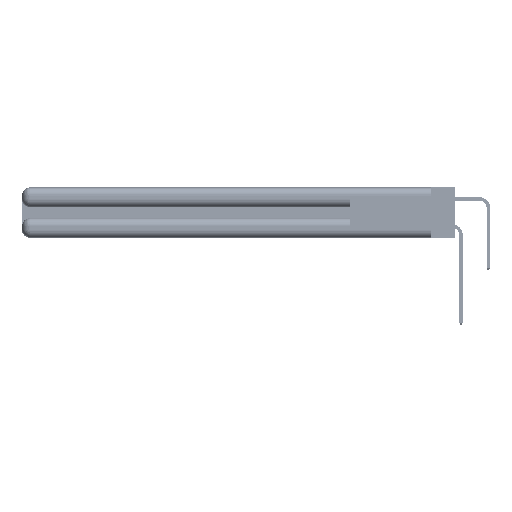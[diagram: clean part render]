
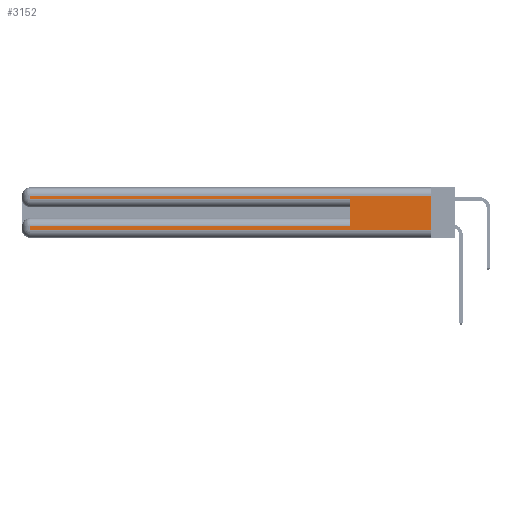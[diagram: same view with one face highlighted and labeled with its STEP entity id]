
A CAD part, left-side view. The second image highlights one B-rep face of the part: STEP entity #3152.
In plain terms, the highlighted planar face has unit normal (-1, 0, 0).
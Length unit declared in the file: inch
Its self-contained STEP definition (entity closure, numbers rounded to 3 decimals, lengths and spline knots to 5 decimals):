
#1266 = CARTESIAN_POINT ( 'NONE',  ( 0., 0., 0.085 ) ) ;
#1455 = VERTEX_POINT ( 'NONE', #17711 ) ;
#2959 = ORIENTED_EDGE ( 'NONE', *, *, #5836, .T. ) ;
#3152 = ADVANCED_FACE ( 'NONE', ( #15812 ), #12290, .F. ) ;
#4773 = ORIENTED_EDGE ( 'NONE', *, *, #14614, .T. ) ;
#5836 = EDGE_CURVE ( 'NONE', #51356, #11922, #20394, .T. ) ;
#5953 = VERTEX_POINT ( 'NONE', #56680 ) ;
#6262 = LINE ( 'NONE', #46348, #47936 ) ;
#6384 = LINE ( 'NONE', #8301, #53842 ) ;
#6420 = DIRECTION ( 'NONE',  ( 0., -1., 0. ) ) ;
#6842 = CARTESIAN_POINT ( 'NONE',  ( 0., 0., 0.06 ) ) ;
#8033 = ORIENTED_EDGE ( 'NONE', *, *, #21354, .F. ) ;
#8156 = ORIENTED_EDGE ( 'NONE', *, *, #21799, .F. ) ;
#8167 = AXIS2_PLACEMENT_3D ( 'NONE', #44431, #55079, #16702 ) ;
#8301 = CARTESIAN_POINT ( 'NONE',  ( 0., 0.6, 0.145 ) ) ;
#9534 = DIRECTION ( 'NONE',  ( 0., 1., 0. ) ) ;
#9538 = CARTESIAN_POINT ( 'NONE',  ( 0., 2.94, 0.37 ) ) ;
#11922 = VERTEX_POINT ( 'NONE', #40987 ) ;
#12290 = PLANE ( 'NONE',  #8167 ) ;
#13290 = LINE ( 'NONE', #29374, #29796 ) ;
#13654 = LINE ( 'NONE', #41084, #37311 ) ;
#14614 = EDGE_CURVE ( 'NONE', #1455, #5953, #6262, .T. ) ;
#15181 = LINE ( 'NONE', #9538, #19472 ) ;
#15812 = FACE_OUTER_BOUND ( 'NONE', #48353, .T. ) ;
#16702 = DIRECTION ( 'NONE',  ( 0., 0., -1. ) ) ;
#17130 = VECTOR ( 'NONE', #6420, 39.37008 ) ;
#17711 = CARTESIAN_POINT ( 'NONE',  ( 0., 0., 0.31 ) ) ;
#19472 = VECTOR ( 'NONE', #55698, 39.37008 ) ;
#19954 = VERTEX_POINT ( 'NONE', #22687 ) ;
#20394 = LINE ( 'NONE', #1266, #59277 ) ;
#20502 = CARTESIAN_POINT ( 'NONE',  ( 0., 0., 0.37 ) ) ;
#21083 = EDGE_CURVE ( 'NONE', #11922, #50777, #13654, .T. ) ;
#21354 = EDGE_CURVE ( 'NONE', #1455, #52335, #27208, .T. ) ;
#21799 = EDGE_CURVE ( 'NONE', #51356, #19954, #6384, .T. ) ;
#22687 = CARTESIAN_POINT ( 'NONE',  ( 0., 0.6, 0.285 ) ) ;
#26573 = VERTEX_POINT ( 'NONE', #51967 ) ;
#27208 = LINE ( 'NONE', #20502, #56703 ) ;
#28840 = EDGE_CURVE ( 'NONE', #5953, #26573, #15181, .T. ) ;
#29374 = CARTESIAN_POINT ( 'NONE',  ( 0., 0., 0.285 ) ) ;
#29796 = VECTOR ( 'NONE', #56725, 39.37008 ) ;
#31964 = ORIENTED_EDGE ( 'NONE', *, *, #21083, .T. ) ;
#32956 = EDGE_CURVE ( 'NONE', #26573, #19954, #13290, .T. ) ;
#33607 = LINE ( 'NONE', #33874, #17130 ) ;
#33874 = CARTESIAN_POINT ( 'NONE',  ( 0., 0., 0.06 ) ) ;
#33948 = DIRECTION ( 'NONE',  ( 0., 0., -1. ) ) ;
#37311 = VECTOR ( 'NONE', #41678, 39.37008 ) ;
#39554 = CARTESIAN_POINT ( 'NONE',  ( 0., 2.94, 0.06 ) ) ;
#39597 = ORIENTED_EDGE ( 'NONE', *, *, #32956, .T. ) ;
#39686 = CARTESIAN_POINT ( 'NONE',  ( 0., 0.6, 0.085 ) ) ;
#40418 = DIRECTION ( 'NONE',  ( 0., 0., 1. ) ) ;
#40987 = CARTESIAN_POINT ( 'NONE',  ( 0., 2.94, 0.085 ) ) ;
#41084 = CARTESIAN_POINT ( 'NONE',  ( 0., 2.94, 0.37 ) ) ;
#41678 = DIRECTION ( 'NONE',  ( 0., 0., -1. ) ) ;
#44431 = CARTESIAN_POINT ( 'NONE',  ( 0., 0., 0.37 ) ) ;
#46348 = CARTESIAN_POINT ( 'NONE',  ( 0., 0., 0.31 ) ) ;
#47936 = VECTOR ( 'NONE', #51349, 39.37008 ) ;
#48353 = EDGE_LOOP ( 'NONE', ( #8033, #4773, #53984, #39597, #8156, #2959, #31964, #49103 ) ) ;
#49103 = ORIENTED_EDGE ( 'NONE', *, *, #50345, .T. ) ;
#50345 = EDGE_CURVE ( 'NONE', #50777, #52335, #33607, .T. ) ;
#50777 = VERTEX_POINT ( 'NONE', #39554 ) ;
#51349 = DIRECTION ( 'NONE',  ( 0., 1., 0. ) ) ;
#51356 = VERTEX_POINT ( 'NONE', #39686 ) ;
#51967 = CARTESIAN_POINT ( 'NONE',  ( 0., 2.94, 0.285 ) ) ;
#52335 = VERTEX_POINT ( 'NONE', #6842 ) ;
#53842 = VECTOR ( 'NONE', #40418, 39.37008 ) ;
#53984 = ORIENTED_EDGE ( 'NONE', *, *, #28840, .T. ) ;
#55079 = DIRECTION ( 'NONE',  ( 1., 0., 0. ) ) ;
#55698 = DIRECTION ( 'NONE',  ( 0., 0., -1. ) ) ;
#56680 = CARTESIAN_POINT ( 'NONE',  ( 0., 2.94, 0.31 ) ) ;
#56703 = VECTOR ( 'NONE', #33948, 39.37008 ) ;
#56725 = DIRECTION ( 'NONE',  ( 0., -1., 0. ) ) ;
#59277 = VECTOR ( 'NONE', #9534, 39.37008 ) ;
